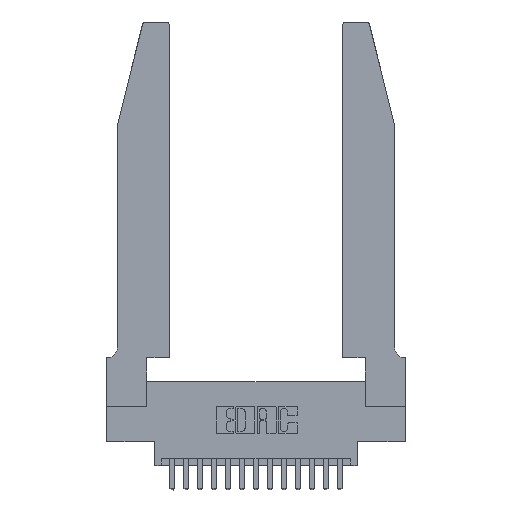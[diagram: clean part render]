
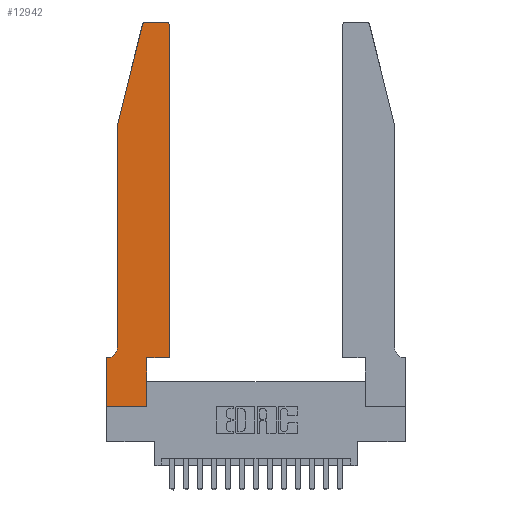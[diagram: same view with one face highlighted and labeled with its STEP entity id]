
A CAD part, top view. The second image highlights one B-rep face of the part: STEP entity #12942.
In plain terms, the highlighted planar face has unit normal (0, 0, 1).
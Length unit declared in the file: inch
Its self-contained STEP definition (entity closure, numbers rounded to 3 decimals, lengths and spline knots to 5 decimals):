
#63 = DIRECTION ( 'NONE',  ( -1., 0., 0. ) ) ;
#210 = ORIENTED_EDGE ( 'NONE', *, *, #368, .T. ) ;
#306 = CARTESIAN_POINT ( 'NONE',  ( 0.2865, 0.35, 0.37 ) ) ;
#368 = EDGE_CURVE ( 'NONE', #8605, #13004, #3533, .T. ) ;
#561 = VERTEX_POINT ( 'NONE', #12124 ) ;
#650 = CARTESIAN_POINT ( 'NONE',  ( 0.4205, 2.72, 0.37 ) ) ;
#773 = PLANE ( 'NONE',  #18568 ) ;
#786 = LINE ( 'NONE', #13367, #6787 ) ;
#817 = VECTOR ( 'NONE', #3120, 39.37008 ) ;
#1108 = CARTESIAN_POINT ( 'NONE',  ( 0.4505, 2.72, 0.37 ) ) ;
#1233 = ORIENTED_EDGE ( 'NONE', *, *, #9559, .T. ) ;
#1285 = VERTEX_POINT ( 'NONE', #4970 ) ;
#1314 = ORIENTED_EDGE ( 'NONE', *, *, #17561, .T. ) ;
#1533 = ORIENTED_EDGE ( 'NONE', *, *, #9385, .T. ) ;
#1707 = CARTESIAN_POINT ( 'NONE',  ( 0.0755, 0.35, 0.37 ) ) ;
#1992 = DIRECTION ( 'NONE',  ( 0., 0., 1. ) ) ;
#2000 = EDGE_CURVE ( 'NONE', #13004, #561, #11321, .T. ) ;
#2064 = DIRECTION ( 'NONE',  ( 0., 0., 1. ) ) ;
#2184 = CARTESIAN_POINT ( 'NONE',  ( 0., 0.35, 0.37 ) ) ;
#2345 = EDGE_CURVE ( 'NONE', #561, #14175, #9034, .T. ) ;
#2476 = DIRECTION ( 'NONE',  ( -0.239, -0.971, 0. ) ) ;
#2897 = VERTEX_POINT ( 'NONE', #17265 ) ;
#2906 = CARTESIAN_POINT ( 'NONE',  ( 0., 0.35, 0.37 ) ) ;
#3120 = DIRECTION ( 'NONE',  ( 0., -1., 0. ) ) ;
#3274 = CARTESIAN_POINT ( 'NONE',  ( 0.4505, 0.35, 0.37 ) ) ;
#3420 = ORIENTED_EDGE ( 'NONE', *, *, #12374, .T. ) ;
#3533 = LINE ( 'NONE', #17180, #4457 ) ;
#3544 = DIRECTION ( 'NONE',  ( 1., 0., 0. ) ) ;
#4305 = DIRECTION ( 'NONE',  ( 0., 0., -1. ) ) ;
#4419 = ORIENTED_EDGE ( 'NONE', *, *, #10686, .T. ) ;
#4457 = VECTOR ( 'NONE', #12830, 39.37008 ) ;
#4516 = LINE ( 'NONE', #13592, #817 ) ;
#4585 = VERTEX_POINT ( 'NONE', #6852 ) ;
#4970 = CARTESIAN_POINT ( 'NONE',  ( 0.2865, 0., 0.37 ) ) ;
#5084 = CARTESIAN_POINT ( 'NONE',  ( 0.0755, 2., 0.37 ) ) ;
#6174 = LINE ( 'NONE', #9853, #12624 ) ;
#6200 = VERTEX_POINT ( 'NONE', #5084 ) ;
#6316 = CIRCLE ( 'NONE', #17744, 0.03 ) ;
#6511 = ORIENTED_EDGE ( 'NONE', *, *, #2000, .T. ) ;
#6640 = EDGE_LOOP ( 'NONE', ( #18974, #17430, #1314, #4419, #3420, #8253, #18450, #1533, #1233, #9210, #210, #6511 ) ) ;
#6787 = VECTOR ( 'NONE', #17876, 39.37008 ) ;
#6852 = CARTESIAN_POINT ( 'NONE',  ( 0., 0., 0.37 ) ) ;
#7095 = VERTEX_POINT ( 'NONE', #2906 ) ;
#7619 = LINE ( 'NONE', #3274, #9223 ) ;
#8253 = ORIENTED_EDGE ( 'NONE', *, *, #8455, .T. ) ;
#8433 = DIRECTION ( 'NONE',  ( 1., 0., 0. ) ) ;
#8455 = EDGE_CURVE ( 'NONE', #15649, #7095, #9836, .T. ) ;
#8605 = VERTEX_POINT ( 'NONE', #16952 ) ;
#8699 = VECTOR ( 'NONE', #10806, 39.37008 ) ;
#8924 = CARTESIAN_POINT ( 'NONE',  ( 0.0055, 0.42, 0.37 ) ) ;
#9030 = CARTESIAN_POINT ( 'NONE',  ( 0.0755, 0.42, 0.37 ) ) ;
#9034 = LINE ( 'NONE', #14916, #18017 ) ;
#9210 = ORIENTED_EDGE ( 'NONE', *, *, #17044, .T. ) ;
#9223 = VECTOR ( 'NONE', #14783, 39.37008 ) ;
#9385 = EDGE_CURVE ( 'NONE', #4585, #1285, #6174, .T. ) ;
#9559 = EDGE_CURVE ( 'NONE', #1285, #11403, #11926, .T. ) ;
#9577 = EDGE_CURVE ( 'NONE', #7095, #4585, #4516, .T. ) ;
#9647 = VERTEX_POINT ( 'NONE', #9030 ) ;
#9671 = DIRECTION ( 'NONE',  ( 1., 0., 0. ) ) ;
#9836 = LINE ( 'NONE', #1707, #8699 ) ;
#9853 = CARTESIAN_POINT ( 'NONE',  ( 0., 0., 0.37 ) ) ;
#10686 = EDGE_CURVE ( 'NONE', #6200, #9647, #786, .T. ) ;
#10806 = DIRECTION ( 'NONE',  ( -1., 0., 0. ) ) ;
#10880 = CARTESIAN_POINT ( 'NONE',  ( 0.0055, 0.35, 0.37 ) ) ;
#10926 = DIRECTION ( 'NONE',  ( 0., 0., 1. ) ) ;
#11021 = EDGE_CURVE ( 'NONE', #14175, #2897, #6316, .T. ) ;
#11321 = CIRCLE ( 'NONE', #14185, 0.03 ) ;
#11403 = VERTEX_POINT ( 'NONE', #12361 ) ;
#11718 = VECTOR ( 'NONE', #2476, 39.37008 ) ;
#11926 = LINE ( 'NONE', #306, #15581 ) ;
#12124 = CARTESIAN_POINT ( 'NONE',  ( 0.4205, 2.75, 0.37 ) ) ;
#12361 = CARTESIAN_POINT ( 'NONE',  ( 0.2865, 0.35, 0.37 ) ) ;
#12374 = EDGE_CURVE ( 'NONE', #9647, #15649, #13427, .T. ) ;
#12624 = VECTOR ( 'NONE', #8433, 39.37008 ) ;
#12830 = DIRECTION ( 'NONE',  ( 0., 1., 0. ) ) ;
#12863 = AXIS2_PLACEMENT_3D ( 'NONE', #8924, #4305, #63 ) ;
#12942 = ADVANCED_FACE ( 'NONE', ( #16389 ), #773, .T. ) ;
#13004 = VERTEX_POINT ( 'NONE', #1108 ) ;
#13305 = CARTESIAN_POINT ( 'NONE',  ( 0.284, 2.75, 0.37 ) ) ;
#13367 = CARTESIAN_POINT ( 'NONE',  ( 0.0755, 2., 0.37 ) ) ;
#13427 = CIRCLE ( 'NONE', #12863, 0.07 ) ;
#13592 = CARTESIAN_POINT ( 'NONE',  ( 0., 0., 0.37 ) ) ;
#14175 = VERTEX_POINT ( 'NONE', #13305 ) ;
#14185 = AXIS2_PLACEMENT_3D ( 'NONE', #650, #2064, #3544 ) ;
#14783 = DIRECTION ( 'NONE',  ( 1., 0., 0. ) ) ;
#14916 = CARTESIAN_POINT ( 'NONE',  ( 0.2605, 2.75, 0.37 ) ) ;
#14982 = DIRECTION ( 'NONE',  ( -1., 0., 0. ) ) ;
#15400 = CARTESIAN_POINT ( 'NONE',  ( 0.284, 2.72, 0.37 ) ) ;
#15581 = VECTOR ( 'NONE', #16481, 39.37008 ) ;
#15649 = VERTEX_POINT ( 'NONE', #10880 ) ;
#15769 = CARTESIAN_POINT ( 'NONE',  ( 0.0755, 2., 0.37 ) ) ;
#16389 = FACE_OUTER_BOUND ( 'NONE', #6640, .T. ) ;
#16481 = DIRECTION ( 'NONE',  ( 0., 1., 0. ) ) ;
#16830 = DIRECTION ( 'NONE',  ( 1., 0., 0. ) ) ;
#16952 = CARTESIAN_POINT ( 'NONE',  ( 0.4505, 0.35, 0.37 ) ) ;
#17044 = EDGE_CURVE ( 'NONE', #11403, #8605, #7619, .T. ) ;
#17180 = CARTESIAN_POINT ( 'NONE',  ( 0.4505, 0.35, 0.37 ) ) ;
#17265 = CARTESIAN_POINT ( 'NONE',  ( 0.25487, 2.72718, 0.37 ) ) ;
#17430 = ORIENTED_EDGE ( 'NONE', *, *, #11021, .T. ) ;
#17561 = EDGE_CURVE ( 'NONE', #2897, #6200, #17966, .T. ) ;
#17744 = AXIS2_PLACEMENT_3D ( 'NONE', #15400, #1992, #9671 ) ;
#17876 = DIRECTION ( 'NONE',  ( 0., -1., 0. ) ) ;
#17966 = LINE ( 'NONE', #15769, #11718 ) ;
#18017 = VECTOR ( 'NONE', #14982, 39.37008 ) ;
#18450 = ORIENTED_EDGE ( 'NONE', *, *, #9577, .T. ) ;
#18568 = AXIS2_PLACEMENT_3D ( 'NONE', #2184, #10926, #16830 ) ;
#18974 = ORIENTED_EDGE ( 'NONE', *, *, #2345, .T. ) ;
